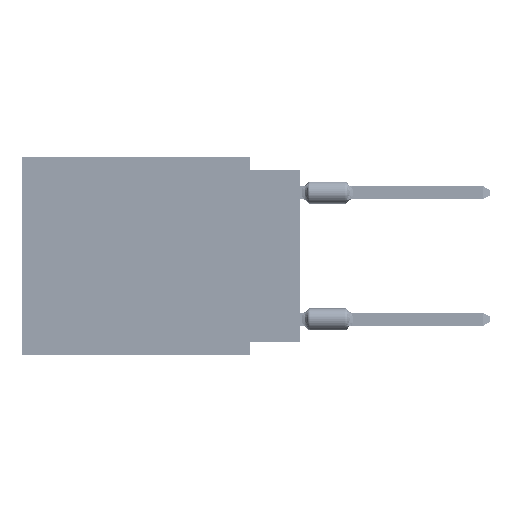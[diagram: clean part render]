
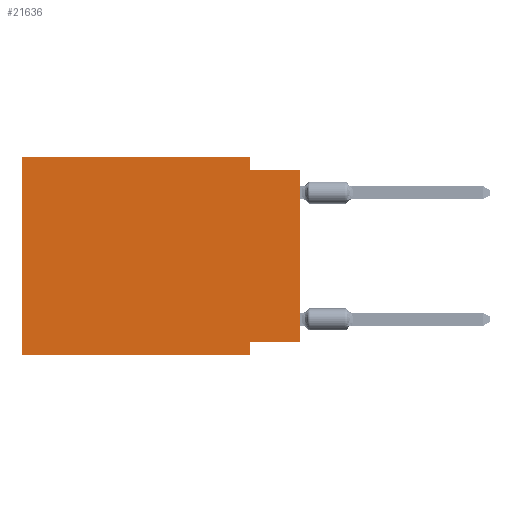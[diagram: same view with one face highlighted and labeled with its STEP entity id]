
A CAD part, left-side view. The second image highlights one B-rep face of the part: STEP entity #21636.
In plain terms, the highlighted planar face has unit normal (-1, 0, 0).
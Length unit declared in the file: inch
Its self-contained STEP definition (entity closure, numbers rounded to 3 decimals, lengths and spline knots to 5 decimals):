
#1726 = DIRECTION ( 'NONE',  ( 0., 0., -1. ) ) ;
#2073 = CARTESIAN_POINT ( 'NONE',  ( 0., 0.55, 0. ) ) ;
#3319 = CARTESIAN_POINT ( 'NONE',  ( 0., 0., -0.365 ) ) ;
#4174 = LINE ( 'NONE', #62155, #34662 ) ;
#5270 = EDGE_CURVE ( 'NONE', #59118, #43353, #66114, .T. ) ;
#6839 = EDGE_CURVE ( 'NONE', #74144, #50908, #54301, .T. ) ;
#9812 = VECTOR ( 'NONE', #36003, 39.37008 ) ;
#10279 = ORIENTED_EDGE ( 'NONE', *, *, #20906, .T. ) ;
#10763 = CARTESIAN_POINT ( 'NONE',  ( 0., 0.1, -0.39 ) ) ;
#12917 = DIRECTION ( 'NONE',  ( 0., -1., 0. ) ) ;
#18437 = ORIENTED_EDGE ( 'NONE', *, *, #5270, .F. ) ;
#19683 = CARTESIAN_POINT ( 'NONE',  ( 0., 0.55, -0.39 ) ) ;
#20906 = EDGE_CURVE ( 'NONE', #59118, #47330, #46153, .T. ) ;
#21364 = VECTOR ( 'NONE', #75028, 39.37008 ) ;
#21636 = ADVANCED_FACE ( 'NONE', ( #24856 ), #76136, .F. ) ;
#22978 = CARTESIAN_POINT ( 'NONE',  ( 0., 0., 0. ) ) ;
#24567 = CARTESIAN_POINT ( 'NONE',  ( 0., 0.55, 0. ) ) ;
#24856 = FACE_OUTER_BOUND ( 'NONE', #35826, .T. ) ;
#30870 = LINE ( 'NONE', #24567, #21364 ) ;
#31539 = EDGE_CURVE ( 'NONE', #32447, #63602, #78914, .T. ) ;
#32447 = VERTEX_POINT ( 'NONE', #41275 ) ;
#32820 = DIRECTION ( 'NONE',  ( 1., 0., 0. ) ) ;
#34610 = EDGE_CURVE ( 'NONE', #50908, #63602, #62539, .T. ) ;
#34662 = VECTOR ( 'NONE', #50366, 39.37008 ) ;
#35826 = EDGE_LOOP ( 'NONE', ( #60351, #48137, #81364, #37858, #18437, #10279, #76226, #48130 ) ) ;
#36003 = DIRECTION ( 'NONE',  ( 0., 0., 1. ) ) ;
#36603 = CARTESIAN_POINT ( 'NONE',  ( 0., 0.1, 0. ) ) ;
#37858 = ORIENTED_EDGE ( 'NONE', *, *, #69193, .F. ) ;
#41275 = CARTESIAN_POINT ( 'NONE',  ( 0., 0., -0.365 ) ) ;
#42175 = EDGE_CURVE ( 'NONE', #69007, #47330, #4174, .T. ) ;
#43353 = VERTEX_POINT ( 'NONE', #2073 ) ;
#43713 = VECTOR ( 'NONE', #71793, 39.37008 ) ;
#46153 = LINE ( 'NONE', #19683, #43713 ) ;
#47330 = VERTEX_POINT ( 'NONE', #10763 ) ;
#47392 = VECTOR ( 'NONE', #61450, 39.37008 ) ;
#48130 = ORIENTED_EDGE ( 'NONE', *, *, #53802, .F. ) ;
#48137 = ORIENTED_EDGE ( 'NONE', *, *, #34610, .F. ) ;
#50366 = DIRECTION ( 'NONE',  ( 0., 0., -1. ) ) ;
#50770 = CARTESIAN_POINT ( 'NONE',  ( 0., 0., -0.025 ) ) ;
#50908 = VERTEX_POINT ( 'NONE', #66431 ) ;
#51567 = CARTESIAN_POINT ( 'NONE',  ( 0., 0.1, -0.365 ) ) ;
#52810 = VECTOR ( 'NONE', #12917, 39.37008 ) ;
#53112 = CARTESIAN_POINT ( 'NONE',  ( 0., 0.1, 0. ) ) ;
#53802 = EDGE_CURVE ( 'NONE', #32447, #69007, #54172, .T. ) ;
#54172 = LINE ( 'NONE', #3319, #61298 ) ;
#54301 = LINE ( 'NONE', #36603, #47392 ) ;
#57249 = AXIS2_PLACEMENT_3D ( 'NONE', #59320, #32820, #1726 ) ;
#59118 = VERTEX_POINT ( 'NONE', #78158 ) ;
#59320 = CARTESIAN_POINT ( 'NONE',  ( 0., 0.55, 0. ) ) ;
#60351 = ORIENTED_EDGE ( 'NONE', *, *, #31539, .T. ) ;
#61298 = VECTOR ( 'NONE', #73501, 39.37008 ) ;
#61450 = DIRECTION ( 'NONE',  ( 0., 0., -1. ) ) ;
#62155 = CARTESIAN_POINT ( 'NONE',  ( 0., 0.1, -0.39 ) ) ;
#62539 = LINE ( 'NONE', #50770, #52810 ) ;
#63602 = VERTEX_POINT ( 'NONE', #71618 ) ;
#66114 = LINE ( 'NONE', #72437, #74039 ) ;
#66431 = CARTESIAN_POINT ( 'NONE',  ( 0., 0.1, -0.025 ) ) ;
#69007 = VERTEX_POINT ( 'NONE', #51567 ) ;
#69193 = EDGE_CURVE ( 'NONE', #43353, #74144, #30870, .T. ) ;
#71618 = CARTESIAN_POINT ( 'NONE',  ( 0., 0., -0.025 ) ) ;
#71793 = DIRECTION ( 'NONE',  ( 0., -1., 0. ) ) ;
#72437 = CARTESIAN_POINT ( 'NONE',  ( 0., 0.55, 0. ) ) ;
#73501 = DIRECTION ( 'NONE',  ( 0., 1., 0. ) ) ;
#74039 = VECTOR ( 'NONE', #79156, 39.37008 ) ;
#74144 = VERTEX_POINT ( 'NONE', #53112 ) ;
#75028 = DIRECTION ( 'NONE',  ( 0., -1., 0. ) ) ;
#76136 = PLANE ( 'NONE',  #57249 ) ;
#76226 = ORIENTED_EDGE ( 'NONE', *, *, #42175, .F. ) ;
#78158 = CARTESIAN_POINT ( 'NONE',  ( 0., 0.55, -0.39 ) ) ;
#78914 = LINE ( 'NONE', #22978, #9812 ) ;
#79156 = DIRECTION ( 'NONE',  ( 0., 0., 1. ) ) ;
#81364 = ORIENTED_EDGE ( 'NONE', *, *, #6839, .F. ) ;
